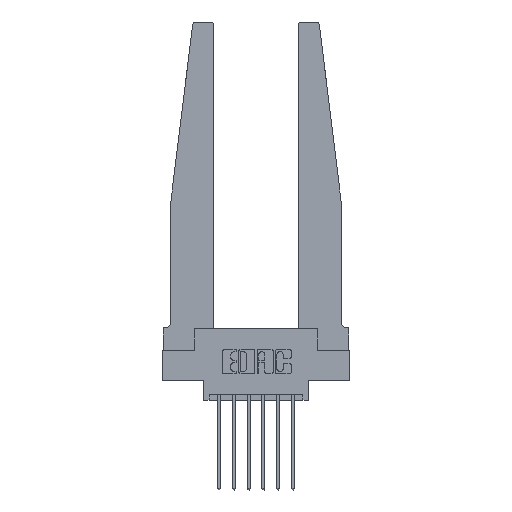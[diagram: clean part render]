
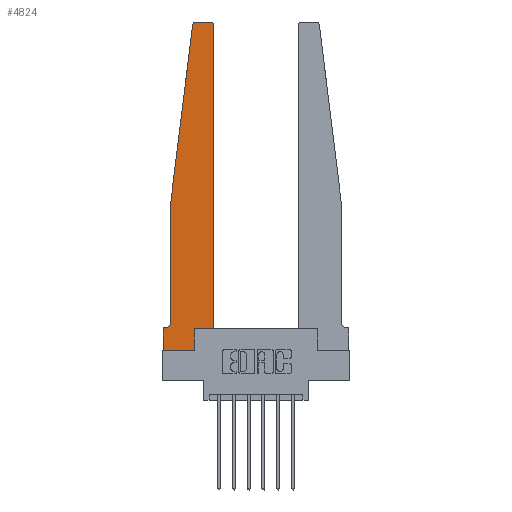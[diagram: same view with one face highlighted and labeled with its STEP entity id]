
A CAD part, top view. The second image highlights one B-rep face of the part: STEP entity #4824.
In plain terms, the highlighted planar face has unit normal (0, 0, 1).
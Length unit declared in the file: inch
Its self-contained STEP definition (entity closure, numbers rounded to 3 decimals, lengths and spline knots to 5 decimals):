
#148 = VECTOR ( 'NONE', #737, 39.37008 ) ;
#189 = CARTESIAN_POINT ( 'NONE',  ( 0.425, 0.18, 0.37 ) ) ;
#316 = VECTOR ( 'NONE', #3562, 39.37008 ) ;
#340 = EDGE_CURVE ( 'NONE', #4011, #3372, #2476, .T. ) ;
#484 = LINE ( 'NONE', #3862, #148 ) ;
#562 = EDGE_CURVE ( 'NONE', #8934, #6492, #484, .T. ) ;
#570 = EDGE_CURVE ( 'NONE', #13319, #5043, #5749, .T. ) ;
#607 = DIRECTION ( 'NONE',  ( -0.122, -0.992, 0. ) ) ;
#672 = CARTESIAN_POINT ( 'NONE',  ( 0.2605, 0.18, 0.37 ) ) ;
#737 = DIRECTION ( 'NONE',  ( 0., -1., 0. ) ) ;
#1087 = VECTOR ( 'NONE', #9251, 39.37008 ) ;
#1330 = EDGE_CURVE ( 'NONE', #5043, #11072, #10164, .T. ) ;
#1465 = LINE ( 'NONE', #4786, #12013 ) ;
#1505 = CARTESIAN_POINT ( 'NONE',  ( 0.425, 0.18, 0.37 ) ) ;
#1819 = ORIENTED_EDGE ( 'NONE', *, *, #6992, .T. ) ;
#2240 = AXIS2_PLACEMENT_3D ( 'NONE', #8984, #2688, #10021 ) ;
#2241 = EDGE_CURVE ( 'NONE', #3372, #4314, #8020, .T. ) ;
#2360 = ORIENTED_EDGE ( 'NONE', *, *, #9908, .T. ) ;
#2476 = LINE ( 'NONE', #4396, #8739 ) ;
#2688 = DIRECTION ( 'NONE',  ( 0., 0., 1. ) ) ;
#2804 = VECTOR ( 'NONE', #8527, 39.37008 ) ;
#2916 = DIRECTION ( 'NONE',  ( 0., 0., -1. ) ) ;
#3077 = CARTESIAN_POINT ( 'NONE',  ( 0.2605, 0.18, 0.37 ) ) ;
#3126 = LINE ( 'NONE', #7449, #2804 ) ;
#3372 = VERTEX_POINT ( 'NONE', #11605 ) ;
#3562 = DIRECTION ( 'NONE',  ( 1., 0., 0. ) ) ;
#3659 = AXIS2_PLACEMENT_3D ( 'NONE', #4798, #12176, #5846 ) ;
#3841 = VERTEX_POINT ( 'NONE', #4022 ) ;
#3862 = CARTESIAN_POINT ( 'NONE',  ( 0.065, 1.25, 0.37 ) ) ;
#3903 = CARTESIAN_POINT ( 'NONE',  ( 0., 0., 0.37 ) ) ;
#3984 = CARTESIAN_POINT ( 'NONE',  ( 0., 0., 0.37 ) ) ;
#4011 = VERTEX_POINT ( 'NONE', #12849 ) ;
#4022 = CARTESIAN_POINT ( 'NONE',  ( 0.425, 2.72, 0.37 ) ) ;
#4206 = VECTOR ( 'NONE', #607, 39.37008 ) ;
#4314 = VERTEX_POINT ( 'NONE', #8320 ) ;
#4373 = ORIENTED_EDGE ( 'NONE', *, *, #562, .T. ) ;
#4396 = CARTESIAN_POINT ( 'NONE',  ( 0.25, 2.75, 0.37 ) ) ;
#4434 = ORIENTED_EDGE ( 'NONE', *, *, #1330, .T. ) ;
#4786 = CARTESIAN_POINT ( 'NONE',  ( 0.425, 0.18, 0.37 ) ) ;
#4798 = CARTESIAN_POINT ( 'NONE',  ( 0., 0.1875, 0.37 ) ) ;
#4802 = CARTESIAN_POINT ( 'NONE',  ( 0.065, 1.25, 0.37 ) ) ;
#4824 = ADVANCED_FACE ( 'NONE', ( #9107 ), #8989, .T. ) ;
#4902 = CIRCLE ( 'NONE', #8933, 0.05 ) ;
#4989 = DIRECTION ( 'NONE',  ( 1., 0., 0. ) ) ;
#5043 = VERTEX_POINT ( 'NONE', #10557 ) ;
#5226 = DIRECTION ( 'NONE',  ( 0., 0., 1. ) ) ;
#5749 = LINE ( 'NONE', #3903, #8235 ) ;
#5839 = DIRECTION ( 'NONE',  ( 0., 1., 0. ) ) ;
#5846 = DIRECTION ( 'NONE',  ( 1., 0., 0. ) ) ;
#6492 = VERTEX_POINT ( 'NONE', #9449 ) ;
#6707 = CIRCLE ( 'NONE', #10326, 0.03 ) ;
#6731 = ORIENTED_EDGE ( 'NONE', *, *, #12646, .T. ) ;
#6744 = CARTESIAN_POINT ( 'NONE',  ( 0.065, 1.25, 0.37 ) ) ;
#6973 = ORIENTED_EDGE ( 'NONE', *, *, #570, .T. ) ;
#6992 = EDGE_CURVE ( 'NONE', #10426, #8529, #3126, .T. ) ;
#7046 = LINE ( 'NONE', #4802, #4206 ) ;
#7368 = VECTOR ( 'NONE', #9373, 39.37008 ) ;
#7449 = CARTESIAN_POINT ( 'NONE',  ( 0.065, 0.1875, 0.37 ) ) ;
#8020 = CIRCLE ( 'NONE', #2240, 0.03 ) ;
#8215 = ORIENTED_EDGE ( 'NONE', *, *, #13201, .T. ) ;
#8235 = VECTOR ( 'NONE', #4989, 39.37008 ) ;
#8320 = CARTESIAN_POINT ( 'NONE',  ( 0.24675, 2.72367, 0.37 ) ) ;
#8527 = DIRECTION ( 'NONE',  ( -1., 0., 0. ) ) ;
#8529 = VERTEX_POINT ( 'NONE', #10140 ) ;
#8739 = VECTOR ( 'NONE', #11800, 39.37008 ) ;
#8933 = AXIS2_PLACEMENT_3D ( 'NONE', #9202, #2916, #10247 ) ;
#8934 = VERTEX_POINT ( 'NONE', #6744 ) ;
#8984 = CARTESIAN_POINT ( 'NONE',  ( 0.27653, 2.72, 0.37 ) ) ;
#8989 = PLANE ( 'NONE',  #3659 ) ;
#9107 = FACE_OUTER_BOUND ( 'NONE', #9343, .T. ) ;
#9202 = CARTESIAN_POINT ( 'NONE',  ( 0.015, 0.2375, 0.37 ) ) ;
#9251 = DIRECTION ( 'NONE',  ( 0., -1., 0. ) ) ;
#9343 = EDGE_LOOP ( 'NONE', ( #11195, #12389, #6731, #4373, #9877, #1819, #2360, #6973, #4434, #12881, #10392, #8215 ) ) ;
#9373 = DIRECTION ( 'NONE',  ( 0., 1., 0. ) ) ;
#9449 = CARTESIAN_POINT ( 'NONE',  ( 0.065, 0.2375, 0.37 ) ) ;
#9593 = CARTESIAN_POINT ( 'NONE',  ( 0., 0., 0.37 ) ) ;
#9877 = ORIENTED_EDGE ( 'NONE', *, *, #13121, .T. ) ;
#9908 = EDGE_CURVE ( 'NONE', #8529, #13319, #11967, .T. ) ;
#10021 = DIRECTION ( 'NONE',  ( 1., 0., 0. ) ) ;
#10140 = CARTESIAN_POINT ( 'NONE',  ( 0., 0.1875, 0.37 ) ) ;
#10164 = LINE ( 'NONE', #3077, #7368 ) ;
#10247 = DIRECTION ( 'NONE',  ( -1., 0., 0. ) ) ;
#10326 = AXIS2_PLACEMENT_3D ( 'NONE', #11550, #5226, #12637 ) ;
#10392 = ORIENTED_EDGE ( 'NONE', *, *, #12182, .T. ) ;
#10426 = VERTEX_POINT ( 'NONE', #11201 ) ;
#10557 = CARTESIAN_POINT ( 'NONE',  ( 0.2605, 0., 0.37 ) ) ;
#10837 = LINE ( 'NONE', #1505, #316 ) ;
#11072 = VERTEX_POINT ( 'NONE', #672 ) ;
#11195 = ORIENTED_EDGE ( 'NONE', *, *, #340, .T. ) ;
#11201 = CARTESIAN_POINT ( 'NONE',  ( 0.015, 0.1875, 0.37 ) ) ;
#11526 = EDGE_CURVE ( 'NONE', #11072, #11980, #10837, .T. ) ;
#11550 = CARTESIAN_POINT ( 'NONE',  ( 0.395, 2.72, 0.37 ) ) ;
#11605 = CARTESIAN_POINT ( 'NONE',  ( 0.27653, 2.75, 0.37 ) ) ;
#11800 = DIRECTION ( 'NONE',  ( -1., 0., 0. ) ) ;
#11967 = LINE ( 'NONE', #3984, #1087 ) ;
#11980 = VERTEX_POINT ( 'NONE', #189 ) ;
#12013 = VECTOR ( 'NONE', #5839, 39.37008 ) ;
#12176 = DIRECTION ( 'NONE',  ( 0., 0., 1. ) ) ;
#12182 = EDGE_CURVE ( 'NONE', #11980, #3841, #1465, .T. ) ;
#12389 = ORIENTED_EDGE ( 'NONE', *, *, #2241, .T. ) ;
#12637 = DIRECTION ( 'NONE',  ( 1., 0., 0. ) ) ;
#12646 = EDGE_CURVE ( 'NONE', #4314, #8934, #7046, .T. ) ;
#12849 = CARTESIAN_POINT ( 'NONE',  ( 0.395, 2.75, 0.37 ) ) ;
#12881 = ORIENTED_EDGE ( 'NONE', *, *, #11526, .T. ) ;
#13121 = EDGE_CURVE ( 'NONE', #6492, #10426, #4902, .T. ) ;
#13201 = EDGE_CURVE ( 'NONE', #3841, #4011, #6707, .T. ) ;
#13319 = VERTEX_POINT ( 'NONE', #9593 ) ;
